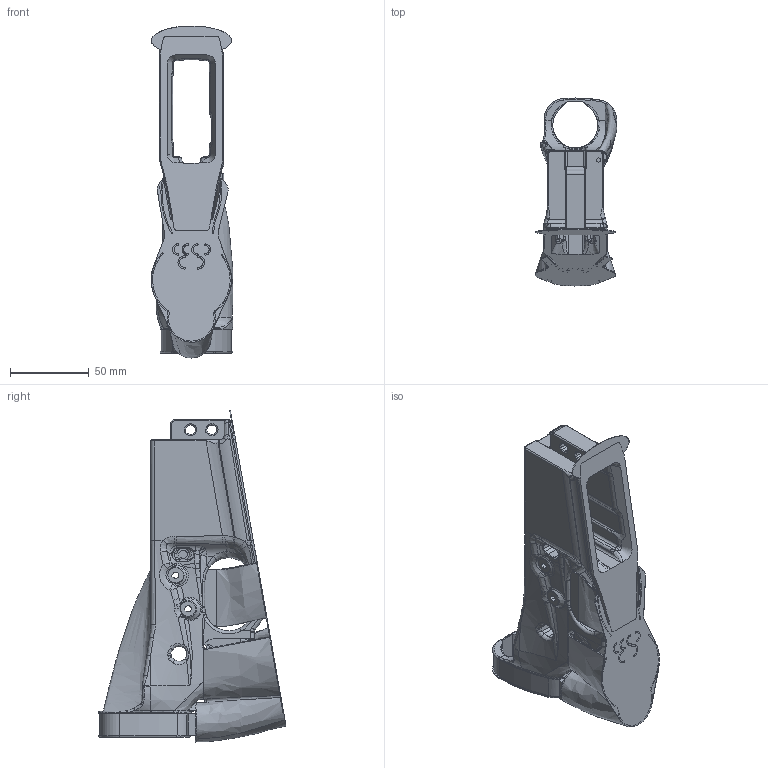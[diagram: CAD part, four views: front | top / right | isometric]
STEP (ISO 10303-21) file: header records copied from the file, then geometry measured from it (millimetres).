
FILE_DESCRIPTION (( 'STEP AP203' ), '1' );
FILE_NAME ('AR-15 SL V3.1 WS.STEP', '2022-05-05T17:09:57', ( '' ), ( '' ), 'SwSTEP 2.0', 'SolidWorks 2021', '' );
FILE_SCHEMA (( 'CONFIG_CONTROL_DESIGN' ));
Products named in the file (1): AR-15 SL V3.1 WS
Bounding box: 51.89 x 119.27 x 210.65 mm (x, y, z)
Volume: 189660.7 mm3; surface area: 98428.8 mm2
Topology: 3 solids, 3 shells, 2098 faces, 5623 edges, 3553 vertices
Faces by surface type: bspline 803, plane 671, cylinder 461, torus 115, cone 32, sphere 16
Entity records: 131706 total; most frequent: CARTESIAN_POINT 85964, ORIENTED_EDGE 11164, DIRECTION 7180, EDGE_CURVE 5582, VERTEX_POINT 3553, AXIS2_PLACEMENT_3D 2453, VECTOR 2274, LINE 2274
